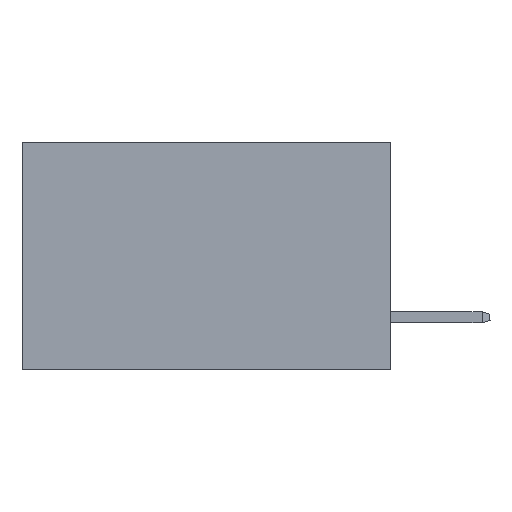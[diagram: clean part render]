
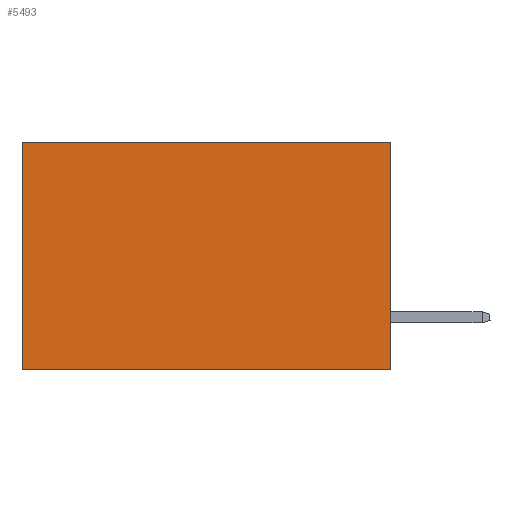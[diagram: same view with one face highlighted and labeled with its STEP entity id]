
A CAD part, left-side view. The second image highlights one B-rep face of the part: STEP entity #5493.
In plain terms, the highlighted planar face has unit normal (-1, 0, 0).
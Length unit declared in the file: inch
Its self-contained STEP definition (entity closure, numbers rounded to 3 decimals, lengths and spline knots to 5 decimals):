
#2411 = CARTESIAN_POINT ( 'NONE',  ( 0.2875, 0.6, 0. ) ) ;
#2458 = VERTEX_POINT ( 'NONE', #22607 ) ;
#2627 = PLANE ( 'NONE',  #2977 ) ;
#2867 = CARTESIAN_POINT ( 'NONE',  ( 0.2875, 0.6, 0. ) ) ;
#2977 = AXIS2_PLACEMENT_3D ( 'NONE', #17191, #6830, #25655 ) ;
#2987 = DIRECTION ( 'NONE',  ( 0., 0., -1. ) ) ;
#3065 = CARTESIAN_POINT ( 'NONE',  ( 0.2875, 0., 0. ) ) ;
#4779 = DIRECTION ( 'NONE',  ( 0., 0., -1. ) ) ;
#5493 = ADVANCED_FACE ( 'NONE', ( #9831 ), #2627, .F. ) ;
#5657 = EDGE_LOOP ( 'NONE', ( #6255, #5939, #17096, #17211 ) ) ;
#5939 = ORIENTED_EDGE ( 'NONE', *, *, #15027, .F. ) ;
#5945 = DIRECTION ( 'NONE',  ( 0., 1., 0. ) ) ;
#6255 = ORIENTED_EDGE ( 'NONE', *, *, #11736, .T. ) ;
#6830 = DIRECTION ( 'NONE',  ( 1., 0., 0. ) ) ;
#6957 = EDGE_CURVE ( 'NONE', #14765, #2458, #13994, .T. ) ;
#7424 = EDGE_CURVE ( 'NONE', #14765, #11869, #14287, .T. ) ;
#7896 = LINE ( 'NONE', #2411, #16018 ) ;
#8449 = VECTOR ( 'NONE', #2987, 39.37008 ) ;
#8657 = VERTEX_POINT ( 'NONE', #25326 ) ;
#9831 = FACE_OUTER_BOUND ( 'NONE', #5657, .T. ) ;
#11248 = VECTOR ( 'NONE', #5945, 39.37008 ) ;
#11736 = EDGE_CURVE ( 'NONE', #11869, #8657, #7896, .T. ) ;
#11869 = VERTEX_POINT ( 'NONE', #2867 ) ;
#13994 = LINE ( 'NONE', #3065, #8449 ) ;
#14287 = LINE ( 'NONE', #23320, #20482 ) ;
#14765 = VERTEX_POINT ( 'NONE', #26760 ) ;
#15027 = EDGE_CURVE ( 'NONE', #2458, #8657, #17417, .T. ) ;
#16018 = VECTOR ( 'NONE', #4779, 39.37008 ) ;
#17096 = ORIENTED_EDGE ( 'NONE', *, *, #6957, .F. ) ;
#17191 = CARTESIAN_POINT ( 'NONE',  ( 0.2875, 0., 0. ) ) ;
#17211 = ORIENTED_EDGE ( 'NONE', *, *, #7424, .T. ) ;
#17417 = LINE ( 'NONE', #18417, #11248 ) ;
#18417 = CARTESIAN_POINT ( 'NONE',  ( 0.2875, 0., -0.37 ) ) ;
#19342 = DIRECTION ( 'NONE',  ( 0., 1., 0. ) ) ;
#20482 = VECTOR ( 'NONE', #19342, 39.37008 ) ;
#22607 = CARTESIAN_POINT ( 'NONE',  ( 0.2875, 0., -0.37 ) ) ;
#23320 = CARTESIAN_POINT ( 'NONE',  ( 0.2875, 0., 0. ) ) ;
#25326 = CARTESIAN_POINT ( 'NONE',  ( 0.2875, 0.6, -0.37 ) ) ;
#25655 = DIRECTION ( 'NONE',  ( 0., 0., -1. ) ) ;
#26760 = CARTESIAN_POINT ( 'NONE',  ( 0.2875, 0., 0. ) ) ;
